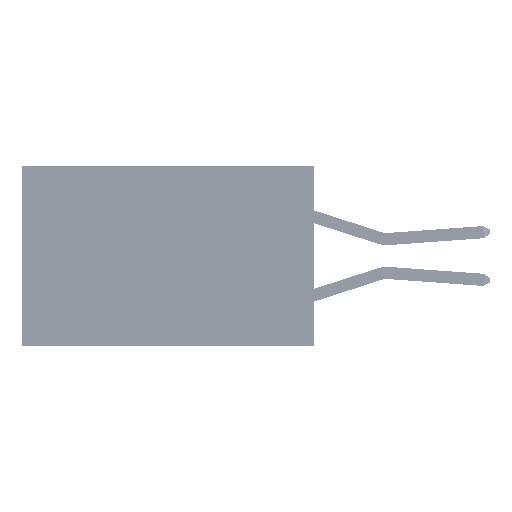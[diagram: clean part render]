
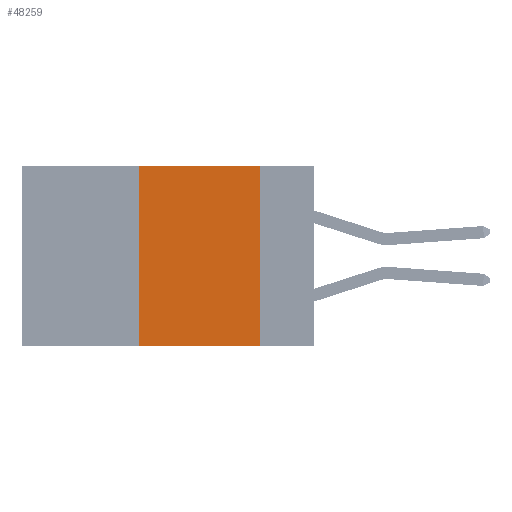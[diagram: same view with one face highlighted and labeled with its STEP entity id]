
A CAD part, left-side view. The second image highlights one B-rep face of the part: STEP entity #48259.
In plain terms, the highlighted planar face has unit normal (-1, 0, 0).
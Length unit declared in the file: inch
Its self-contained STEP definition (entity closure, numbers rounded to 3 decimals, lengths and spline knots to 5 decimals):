
#1580 = EDGE_CURVE ( 'NONE', #34849, #43394, #33781, .T. ) ;
#3523 = CARTESIAN_POINT ( 'NONE',  ( 0., 0.36, -0.37 ) ) ;
#3739 = DIRECTION ( 'NONE',  ( 0., -1., 0. ) ) ;
#4700 = CARTESIAN_POINT ( 'NONE',  ( 0., 0.11, -0.37 ) ) ;
#6147 = VECTOR ( 'NONE', #32464, 39.37008 ) ;
#6965 = EDGE_CURVE ( 'NONE', #39271, #43394, #37869, .T. ) ;
#7685 = VECTOR ( 'NONE', #13816, 39.37008 ) ;
#8200 = AXIS2_PLACEMENT_3D ( 'NONE', #15944, #27666, #42864 ) ;
#12571 = ORIENTED_EDGE ( 'NONE', *, *, #24827, .F. ) ;
#13816 = DIRECTION ( 'NONE',  ( 0., 0., 1. ) ) ;
#14537 = CARTESIAN_POINT ( 'NONE',  ( 0., 0.36, 0. ) ) ;
#15939 = EDGE_LOOP ( 'NONE', ( #16498, #18746, #12571, #34690 ) ) ;
#15944 = CARTESIAN_POINT ( 'NONE',  ( 0., 0.6, 0. ) ) ;
#16498 = ORIENTED_EDGE ( 'NONE', *, *, #1580, .F. ) ;
#16995 = CARTESIAN_POINT ( 'NONE',  ( 0., 0.6, 0. ) ) ;
#18746 = ORIENTED_EDGE ( 'NONE', *, *, #29609, .F. ) ;
#19442 = FACE_OUTER_BOUND ( 'NONE', #15939, .T. ) ;
#22801 = DIRECTION ( 'NONE',  ( 0., 0., -1. ) ) ;
#23539 = VERTEX_POINT ( 'NONE', #27768 ) ;
#23674 = PLANE ( 'NONE',  #8200 ) ;
#24827 = EDGE_CURVE ( 'NONE', #39271, #23539, #25503, .T. ) ;
#25158 = VECTOR ( 'NONE', #22801, 39.37008 ) ;
#25503 = LINE ( 'NONE', #14537, #7685 ) ;
#26324 = CARTESIAN_POINT ( 'NONE',  ( 0., 0.11, 0. ) ) ;
#26535 = CARTESIAN_POINT ( 'NONE',  ( 0., 0.11, 0. ) ) ;
#27666 = DIRECTION ( 'NONE',  ( 1., 0., 0. ) ) ;
#27768 = CARTESIAN_POINT ( 'NONE',  ( 0., 0.36, 0. ) ) ;
#29609 = EDGE_CURVE ( 'NONE', #23539, #34849, #32208, .T. ) ;
#32208 = LINE ( 'NONE', #16995, #6147 ) ;
#32464 = DIRECTION ( 'NONE',  ( 0., -1., 0. ) ) ;
#33781 = LINE ( 'NONE', #26535, #25158 ) ;
#34690 = ORIENTED_EDGE ( 'NONE', *, *, #6965, .T. ) ;
#34849 = VERTEX_POINT ( 'NONE', #26324 ) ;
#35216 = VECTOR ( 'NONE', #3739, 39.37008 ) ;
#35294 = CARTESIAN_POINT ( 'NONE',  ( 0., 0.6, -0.37 ) ) ;
#37869 = LINE ( 'NONE', #35294, #35216 ) ;
#39271 = VERTEX_POINT ( 'NONE', #3523 ) ;
#42864 = DIRECTION ( 'NONE',  ( 0., 0., -1. ) ) ;
#43394 = VERTEX_POINT ( 'NONE', #4700 ) ;
#48259 = ADVANCED_FACE ( 'NONE', ( #19442 ), #23674, .F. ) ;
